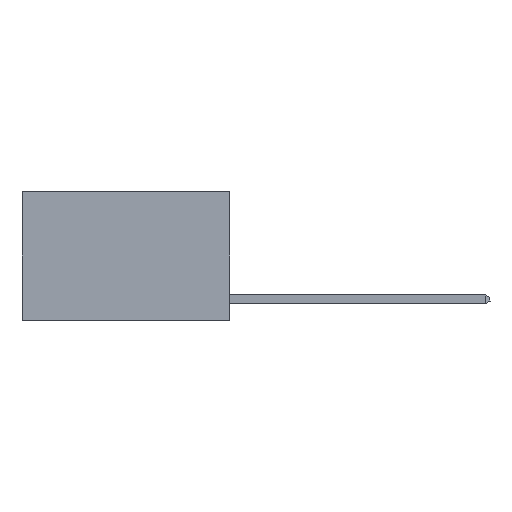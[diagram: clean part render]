
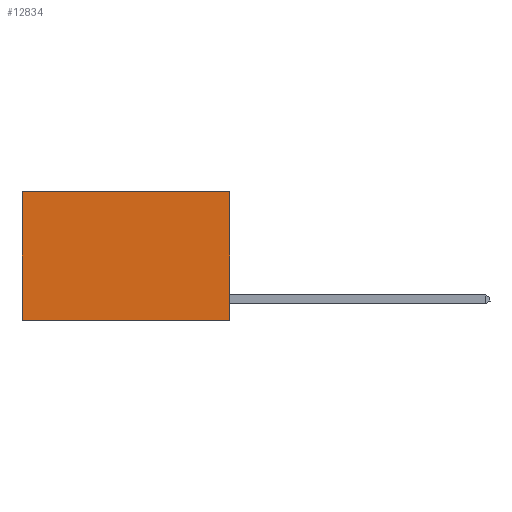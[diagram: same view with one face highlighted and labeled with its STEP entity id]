
A CAD part, left-side view. The second image highlights one B-rep face of the part: STEP entity #12834.
In plain terms, the highlighted planar face has unit normal (-1, 0, 0).
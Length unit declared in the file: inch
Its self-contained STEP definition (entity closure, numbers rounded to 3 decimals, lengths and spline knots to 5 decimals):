
#167 = LINE ( 'NONE', #3018, #8455 ) ;
#199 = VERTEX_POINT ( 'NONE', #228 ) ;
#228 = CARTESIAN_POINT ( 'NONE',  ( 0.2625, 0.6, -0.37 ) ) ;
#590 = CARTESIAN_POINT ( 'NONE',  ( 0.2625, 0., 0. ) ) ;
#1243 = DIRECTION ( 'NONE',  ( 0., 1., 0. ) ) ;
#1642 = DIRECTION ( 'NONE',  ( 0., 0., -1. ) ) ;
#1663 = EDGE_CURVE ( 'NONE', #11071, #199, #4458, .T. ) ;
#1989 = CARTESIAN_POINT ( 'NONE',  ( 0.2625, 0., -0.37 ) ) ;
#2451 = LINE ( 'NONE', #6378, #12867 ) ;
#2492 = DIRECTION ( 'NONE',  ( 0., 0., -1. ) ) ;
#3018 = CARTESIAN_POINT ( 'NONE',  ( 0.2625, 0.6, 0. ) ) ;
#3512 = CARTESIAN_POINT ( 'NONE',  ( 0.2625, 0., 0. ) ) ;
#3713 = CARTESIAN_POINT ( 'NONE',  ( 0.2625, 0., 0. ) ) ;
#4107 = VECTOR ( 'NONE', #2492, 39.37008 ) ;
#4409 = ORIENTED_EDGE ( 'NONE', *, *, #11456, .F. ) ;
#4458 = LINE ( 'NONE', #1989, #7572 ) ;
#6226 = ORIENTED_EDGE ( 'NONE', *, *, #11792, .T. ) ;
#6378 = CARTESIAN_POINT ( 'NONE',  ( 0.2625, 0., 0. ) ) ;
#6813 = PLANE ( 'NONE',  #10906 ) ;
#6926 = DIRECTION ( 'NONE',  ( 0., 1., 0. ) ) ;
#7572 = VECTOR ( 'NONE', #6926, 39.37008 ) ;
#7851 = DIRECTION ( 'NONE',  ( 1., 0., 0. ) ) ;
#8163 = CARTESIAN_POINT ( 'NONE',  ( 0.2625, 0.6, 0. ) ) ;
#8226 = DIRECTION ( 'NONE',  ( 0., 0., -1. ) ) ;
#8455 = VECTOR ( 'NONE', #8226, 39.37008 ) ;
#8508 = VERTEX_POINT ( 'NONE', #8163 ) ;
#8766 = EDGE_LOOP ( 'NONE', ( #6226, #11023, #4409, #10614 ) ) ;
#8911 = VERTEX_POINT ( 'NONE', #3713 ) ;
#9053 = FACE_OUTER_BOUND ( 'NONE', #8766, .T. ) ;
#9342 = EDGE_CURVE ( 'NONE', #8911, #8508, #2451, .T. ) ;
#9536 = LINE ( 'NONE', #3512, #4107 ) ;
#10614 = ORIENTED_EDGE ( 'NONE', *, *, #9342, .T. ) ;
#10906 = AXIS2_PLACEMENT_3D ( 'NONE', #590, #7851, #1642 ) ;
#11023 = ORIENTED_EDGE ( 'NONE', *, *, #1663, .F. ) ;
#11071 = VERTEX_POINT ( 'NONE', #13031 ) ;
#11456 = EDGE_CURVE ( 'NONE', #8911, #11071, #9536, .T. ) ;
#11792 = EDGE_CURVE ( 'NONE', #8508, #199, #167, .T. ) ;
#12834 = ADVANCED_FACE ( 'NONE', ( #9053 ), #6813, .F. ) ;
#12867 = VECTOR ( 'NONE', #1243, 39.37008 ) ;
#13031 = CARTESIAN_POINT ( 'NONE',  ( 0.2625, 0., -0.37 ) ) ;
